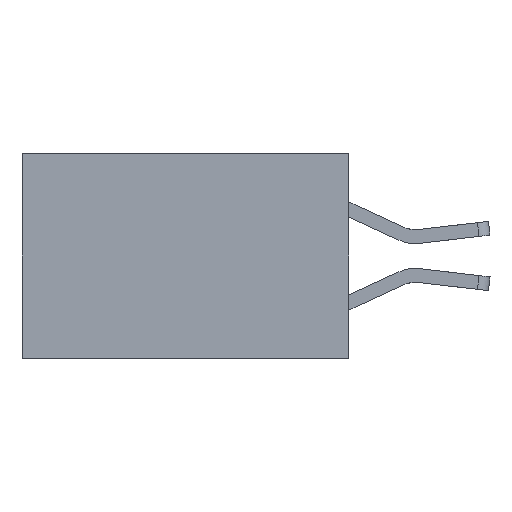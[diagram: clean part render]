
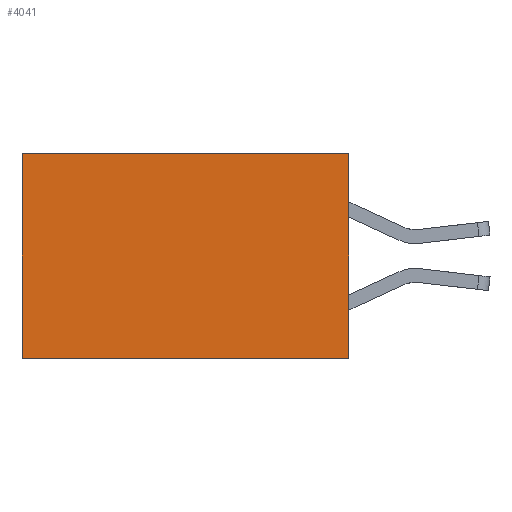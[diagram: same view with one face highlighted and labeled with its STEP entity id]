
A CAD part, left-side view. The second image highlights one B-rep face of the part: STEP entity #4041.
In plain terms, the highlighted planar face has unit normal (-1, 0, 0).
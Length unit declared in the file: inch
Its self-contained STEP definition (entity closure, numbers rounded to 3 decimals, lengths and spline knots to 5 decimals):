
#4 = VERTEX_POINT ( 'NONE', #8922 ) ;
#278 = LINE ( 'NONE', #6095, #1812 ) ;
#346 = VERTEX_POINT ( 'NONE', #3739 ) ;
#355 = DIRECTION ( 'NONE',  ( 0., 0., -1. ) ) ;
#929 = CARTESIAN_POINT ( 'NONE',  ( 0.277, 0.59, -0.37 ) ) ;
#1001 = VECTOR ( 'NONE', #8687, 39.37008 ) ;
#1219 = EDGE_CURVE ( 'NONE', #346, #3013, #10291, .T. ) ;
#1227 = ORIENTED_EDGE ( 'NONE', *, *, #2614, .T. ) ;
#1382 = DIRECTION ( 'NONE',  ( 0., 1., 0. ) ) ;
#1535 = ORIENTED_EDGE ( 'NONE', *, *, #9451, .F. ) ;
#1812 = VECTOR ( 'NONE', #4823, 39.37008 ) ;
#2265 = PLANE ( 'NONE',  #7828 ) ;
#2429 = ORIENTED_EDGE ( 'NONE', *, *, #8582, .T. ) ;
#2614 = EDGE_CURVE ( 'NONE', #9806, #4, #278, .T. ) ;
#2735 = CARTESIAN_POINT ( 'NONE',  ( 0.277, 0., -0.37 ) ) ;
#2833 = DIRECTION ( 'NONE',  ( 1., 0., 0. ) ) ;
#3013 = VERTEX_POINT ( 'NONE', #929 ) ;
#3629 = VECTOR ( 'NONE', #355, 39.37008 ) ;
#3639 = CARTESIAN_POINT ( 'NONE',  ( 0.277, 0.59, -0.37 ) ) ;
#3739 = CARTESIAN_POINT ( 'NONE',  ( 0.277, 0., -0.37 ) ) ;
#4041 = ADVANCED_FACE ( 'NONE', ( #5050 ), #2265, .F. ) ;
#4060 = DIRECTION ( 'NONE',  ( 0., 0., -1. ) ) ;
#4339 = ORIENTED_EDGE ( 'NONE', *, *, #1219, .F. ) ;
#4823 = DIRECTION ( 'NONE',  ( 0., 1., 0. ) ) ;
#5050 = FACE_OUTER_BOUND ( 'NONE', #7918, .T. ) ;
#5889 = LINE ( 'NONE', #10499, #3629 ) ;
#5904 = VECTOR ( 'NONE', #1382, 39.37008 ) ;
#6095 = CARTESIAN_POINT ( 'NONE',  ( 0.277, 0., 0. ) ) ;
#7735 = CARTESIAN_POINT ( 'NONE',  ( 0.277, 0., 0. ) ) ;
#7828 = AXIS2_PLACEMENT_3D ( 'NONE', #2735, #2833, #4060 ) ;
#7918 = EDGE_LOOP ( 'NONE', ( #2429, #4339, #1535, #1227 ) ) ;
#8582 = EDGE_CURVE ( 'NONE', #4, #3013, #10051, .T. ) ;
#8687 = DIRECTION ( 'NONE',  ( 0., 0., -1. ) ) ;
#8922 = CARTESIAN_POINT ( 'NONE',  ( 0.277, 0.59, 0. ) ) ;
#9451 = EDGE_CURVE ( 'NONE', #9806, #346, #5889, .T. ) ;
#9806 = VERTEX_POINT ( 'NONE', #7735 ) ;
#10051 = LINE ( 'NONE', #3639, #1001 ) ;
#10291 = LINE ( 'NONE', #10600, #5904 ) ;
#10499 = CARTESIAN_POINT ( 'NONE',  ( 0.277, 0., -0.37 ) ) ;
#10600 = CARTESIAN_POINT ( 'NONE',  ( 0.277, 0., -0.37 ) ) ;
